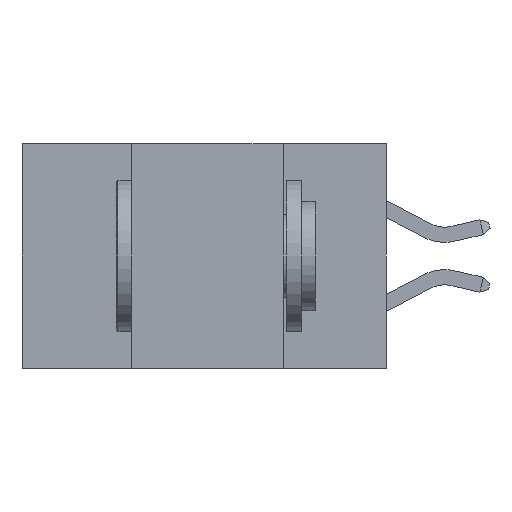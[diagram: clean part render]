
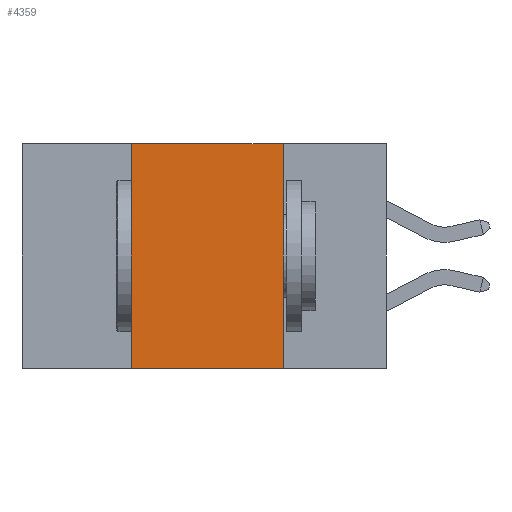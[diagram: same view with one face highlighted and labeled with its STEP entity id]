
A CAD part, left-side view. The second image highlights one B-rep face of the part: STEP entity #4359.
In plain terms, the highlighted planar face has unit normal (-1, 0, 0).
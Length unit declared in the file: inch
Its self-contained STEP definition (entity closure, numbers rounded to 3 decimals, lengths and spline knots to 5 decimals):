
#999 = DIRECTION ( 'NONE',  ( 0., 0., 1. ) ) ;
#2223 = LINE ( 'NONE', #15110, #25381 ) ;
#2285 = CARTESIAN_POINT ( 'NONE',  ( 0., 0.6, -0.37 ) ) ;
#2375 = LINE ( 'NONE', #27871, #26919 ) ;
#3464 = VERTEX_POINT ( 'NONE', #21895 ) ;
#4359 = ADVANCED_FACE ( 'NONE', ( #17734 ), #9119, .F. ) ;
#4563 = DIRECTION ( 'NONE',  ( 0., -1., 0. ) ) ;
#5430 = DIRECTION ( 'NONE',  ( 0., 0., -1. ) ) ;
#5818 = ORIENTED_EDGE ( 'NONE', *, *, #24138, .F. ) ;
#8360 = DIRECTION ( 'NONE',  ( 0., -1., 0. ) ) ;
#9119 = PLANE ( 'NONE',  #13301 ) ;
#9364 = ORIENTED_EDGE ( 'NONE', *, *, #17643, .T. ) ;
#9432 = VECTOR ( 'NONE', #4563, 39.37008 ) ;
#10577 = CARTESIAN_POINT ( 'NONE',  ( 0., 0.17, 0. ) ) ;
#11489 = CARTESIAN_POINT ( 'NONE',  ( 0., 0.6, 0. ) ) ;
#11926 = CARTESIAN_POINT ( 'NONE',  ( 0., 0.42, 0. ) ) ;
#13195 = ORIENTED_EDGE ( 'NONE', *, *, #17943, .F. ) ;
#13301 = AXIS2_PLACEMENT_3D ( 'NONE', #11489, #13331, #19996 ) ;
#13331 = DIRECTION ( 'NONE',  ( 1., 0., 0. ) ) ;
#13954 = LINE ( 'NONE', #2285, #9432 ) ;
#15110 = CARTESIAN_POINT ( 'NONE',  ( 0., 0.6, 0. ) ) ;
#15907 = VERTEX_POINT ( 'NONE', #25253 ) ;
#16700 = ORIENTED_EDGE ( 'NONE', *, *, #28900, .F. ) ;
#17643 = EDGE_CURVE ( 'NONE', #15907, #3464, #13954, .T. ) ;
#17734 = FACE_OUTER_BOUND ( 'NONE', #23628, .T. ) ;
#17943 = EDGE_CURVE ( 'NONE', #15907, #28200, #2375, .T. ) ;
#18812 = CARTESIAN_POINT ( 'NONE',  ( 0., 0.17, 0. ) ) ;
#19996 = DIRECTION ( 'NONE',  ( 0., 0., -1. ) ) ;
#20771 = LINE ( 'NONE', #18812, #28862 ) ;
#21895 = CARTESIAN_POINT ( 'NONE',  ( 0., 0.17, -0.37 ) ) ;
#23628 = EDGE_LOOP ( 'NONE', ( #16700, #5818, #13195, #9364 ) ) ;
#24138 = EDGE_CURVE ( 'NONE', #28200, #27824, #2223, .T. ) ;
#25253 = CARTESIAN_POINT ( 'NONE',  ( 0., 0.42, -0.37 ) ) ;
#25381 = VECTOR ( 'NONE', #8360, 39.37008 ) ;
#26919 = VECTOR ( 'NONE', #999, 39.37008 ) ;
#27824 = VERTEX_POINT ( 'NONE', #10577 ) ;
#27871 = CARTESIAN_POINT ( 'NONE',  ( 0., 0.42, 0. ) ) ;
#28200 = VERTEX_POINT ( 'NONE', #11926 ) ;
#28862 = VECTOR ( 'NONE', #5430, 39.37008 ) ;
#28900 = EDGE_CURVE ( 'NONE', #27824, #3464, #20771, .T. ) ;
